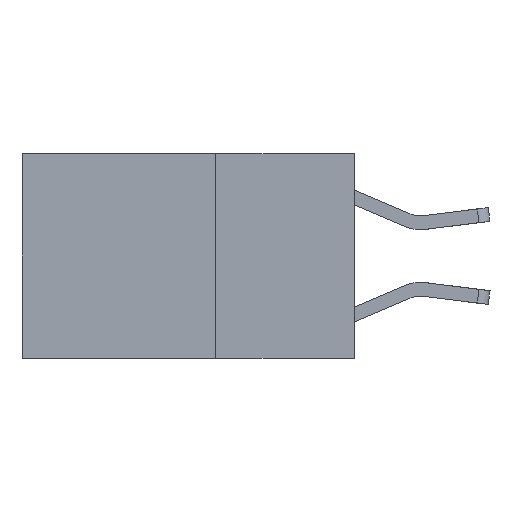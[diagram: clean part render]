
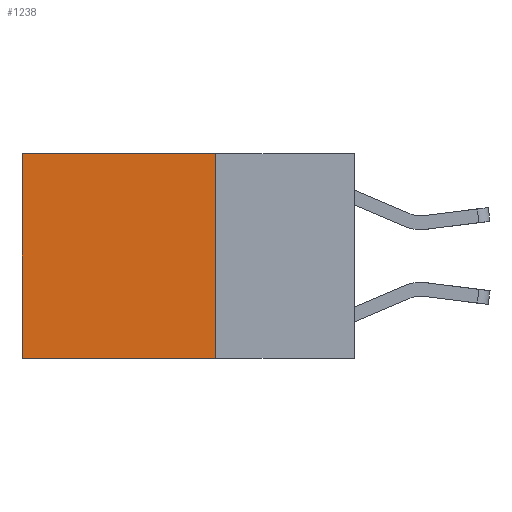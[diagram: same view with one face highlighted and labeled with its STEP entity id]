
A CAD part, left-side view. The second image highlights one B-rep face of the part: STEP entity #1238.
In plain terms, the highlighted planar face has unit normal (-1, 0, 0).
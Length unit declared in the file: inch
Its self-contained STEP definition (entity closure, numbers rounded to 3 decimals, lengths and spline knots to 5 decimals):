
#241 = VECTOR ( 'NONE', #6715, 39.37008 ) ;
#1147 = ORIENTED_EDGE ( 'NONE', *, *, #10873, .T. ) ;
#1238 = ADVANCED_FACE ( 'NONE', ( #8746 ), #11232, .F. ) ;
#1933 = VERTEX_POINT ( 'NONE', #7219 ) ;
#2191 = VERTEX_POINT ( 'NONE', #10687 ) ;
#2413 = CARTESIAN_POINT ( 'NONE',  ( 0.2625, 0.25, -0.37 ) ) ;
#3413 = ORIENTED_EDGE ( 'NONE', *, *, #5608, .F. ) ;
#3535 = LINE ( 'NONE', #2413, #8940 ) ;
#4143 = DIRECTION ( 'NONE',  ( 1., 0., 0. ) ) ;
#4144 = VERTEX_POINT ( 'NONE', #7355 ) ;
#4178 = EDGE_LOOP ( 'NONE', ( #7597, #4684, #3413, #1147 ) ) ;
#4684 = ORIENTED_EDGE ( 'NONE', *, *, #6335, .F. ) ;
#4830 = VERTEX_POINT ( 'NONE', #5690 ) ;
#5457 = CARTESIAN_POINT ( 'NONE',  ( 0.2625, 0.25, 0. ) ) ;
#5584 = CARTESIAN_POINT ( 'NONE',  ( 0.2625, 0.6, 0. ) ) ;
#5608 = EDGE_CURVE ( 'NONE', #4144, #1933, #9115, .T. ) ;
#5690 = CARTESIAN_POINT ( 'NONE',  ( 0.2625, 0.6, 0. ) ) ;
#6327 = LINE ( 'NONE', #10290, #241 ) ;
#6335 = EDGE_CURVE ( 'NONE', #1933, #2191, #3535, .T. ) ;
#6484 = DIRECTION ( 'NONE',  ( 0., 0., -1. ) ) ;
#6715 = DIRECTION ( 'NONE',  ( 0., 1., 0. ) ) ;
#6936 = VECTOR ( 'NONE', #6484, 39.37008 ) ;
#7062 = DIRECTION ( 'NONE',  ( 0., 0., -1. ) ) ;
#7219 = CARTESIAN_POINT ( 'NONE',  ( 0.2625, 0.25, -0.37 ) ) ;
#7355 = CARTESIAN_POINT ( 'NONE',  ( 0.2625, 0.25, 0. ) ) ;
#7473 = EDGE_CURVE ( 'NONE', #4830, #2191, #9381, .T. ) ;
#7597 = ORIENTED_EDGE ( 'NONE', *, *, #7473, .T. ) ;
#7992 = CARTESIAN_POINT ( 'NONE',  ( 0.2625, 0.25, 0. ) ) ;
#8746 = FACE_OUTER_BOUND ( 'NONE', #4178, .T. ) ;
#8770 = DIRECTION ( 'NONE',  ( 0., 1., 0. ) ) ;
#8940 = VECTOR ( 'NONE', #8770, 39.37008 ) ;
#9115 = LINE ( 'NONE', #7992, #9810 ) ;
#9357 = AXIS2_PLACEMENT_3D ( 'NONE', #5457, #4143, #7062 ) ;
#9381 = LINE ( 'NONE', #5584, #6936 ) ;
#9810 = VECTOR ( 'NONE', #10824, 39.37008 ) ;
#10290 = CARTESIAN_POINT ( 'NONE',  ( 0.2625, 0.25, 0. ) ) ;
#10687 = CARTESIAN_POINT ( 'NONE',  ( 0.2625, 0.6, -0.37 ) ) ;
#10824 = DIRECTION ( 'NONE',  ( 0., 0., -1. ) ) ;
#10873 = EDGE_CURVE ( 'NONE', #4144, #4830, #6327, .T. ) ;
#11232 = PLANE ( 'NONE',  #9357 ) ;
